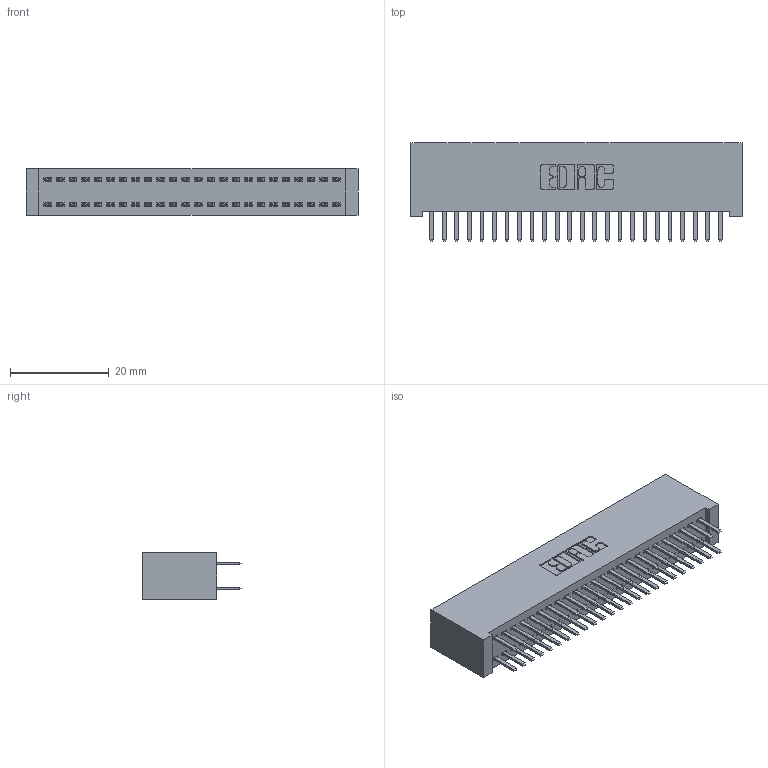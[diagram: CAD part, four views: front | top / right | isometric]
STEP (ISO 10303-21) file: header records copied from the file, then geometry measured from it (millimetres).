
FILE_DESCRIPTION (( 'STEP AP203' ), '1' );
FILE_NAME ('392-048-520-201.STEP', '2019-10-08T00:42:01', ( '' ), ( '' ), 'SwSTEP 2.0', 'SolidWorks 2016', '' );
FILE_SCHEMA (( 'CONFIG_CONTROL_DESIGN' ));
Length unit declared in the file: inch
Products named in the file (3): 392-048-520-201; 342 Part_Lugless; 345-292-001_345-293-120
Assembly tree (49 placements, depth 2):
  392-048-520-201
    342 Part_Lugless
    345-292-001_345-293-120  x48
Bounding box: 67.21 x 20.02 x 9.4 mm (x, y, z)
Volume: 6371.9 mm3; surface area: 10324.7 mm2
Topology: 49 solids, 49 shells, 2790 faces, 8099 edges, 5270 vertices
Faces by surface type: plane 1886, cylinder 904
Entity records: 17473 total; most frequent: CARTESIAN_POINT 2926, ORIENTED_EDGE 2850, DIRECTION 2513, EDGE_CURVE 1425, LINE 1301, VECTOR 1301, VERTEX_POINT 946, AXIS2_PLACEMENT_3D 606
